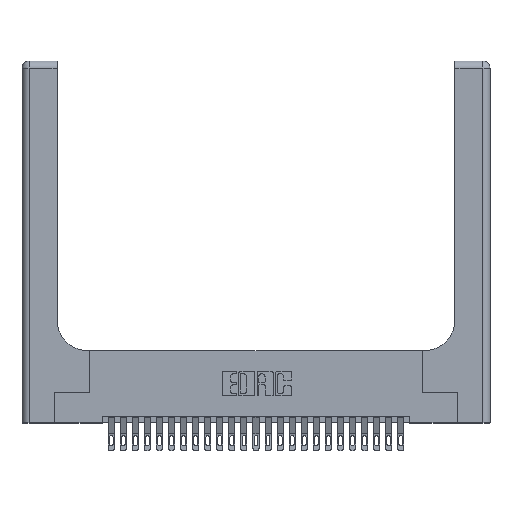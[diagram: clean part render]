
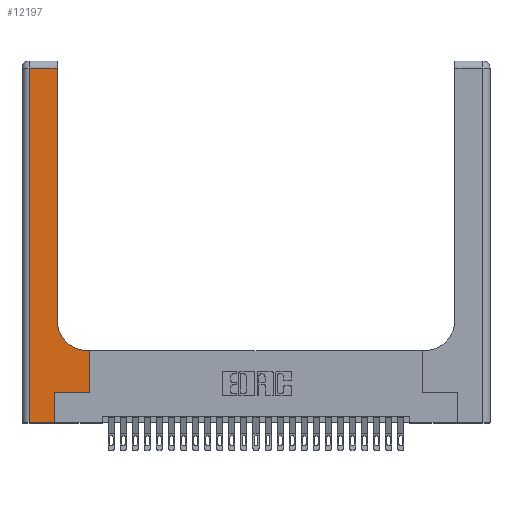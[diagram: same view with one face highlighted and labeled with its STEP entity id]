
A CAD part, top view. The second image highlights one B-rep face of the part: STEP entity #12197.
In plain terms, the highlighted planar face has unit normal (0, 0, 1).
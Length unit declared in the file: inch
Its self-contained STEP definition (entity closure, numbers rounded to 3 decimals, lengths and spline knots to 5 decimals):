
#12 = LINE ( 'NONE', #9352, #11336 ) ;
#282 = VERTEX_POINT ( 'NONE', #26497 ) ;
#387 = VERTEX_POINT ( 'NONE', #24511 ) ;
#941 = LINE ( 'NONE', #19317, #22839 ) ;
#1258 = DIRECTION ( 'NONE',  ( 0., 1., 0. ) ) ;
#1952 = ORIENTED_EDGE ( 'NONE', *, *, #21478, .T. ) ;
#2163 = VERTEX_POINT ( 'NONE', #24411 ) ;
#2564 = VECTOR ( 'NONE', #19264, 39.37008 ) ;
#2626 = CARTESIAN_POINT ( 'NONE',  ( 0.5585, 0.25, 0.37 ) ) ;
#2942 = EDGE_CURVE ( 'NONE', #15907, #387, #3555, .T. ) ;
#3529 = FACE_OUTER_BOUND ( 'NONE', #6134, .T. ) ;
#3555 = LINE ( 'NONE', #5350, #25381 ) ;
#3819 = CIRCLE ( 'NONE', #7777, 0.25 ) ;
#4368 = EDGE_CURVE ( 'NONE', #282, #26265, #15913, .T. ) ;
#5350 = CARTESIAN_POINT ( 'NONE',  ( 0.2915, 3., 0.37 ) ) ;
#5455 = CARTESIAN_POINT ( 'NONE',  ( 0., 2.94, 0.37 ) ) ;
#5601 = ORIENTED_EDGE ( 'NONE', *, *, #16830, .T. ) ;
#5917 = AXIS2_PLACEMENT_3D ( 'NONE', #23738, #25823, #13221 ) ;
#6134 = EDGE_LOOP ( 'NONE', ( #17461, #24082, #26692, #8557, #19874, #5601, #1952, #10276, #25451 ) ) ;
#7440 = DIRECTION ( 'NONE',  ( 1., 0., 0. ) ) ;
#7510 = CARTESIAN_POINT ( 'NONE',  ( 0.5415, 0.85, 0.37 ) ) ;
#7777 = AXIS2_PLACEMENT_3D ( 'NONE', #7510, #22324, #9649 ) ;
#7861 = CARTESIAN_POINT ( 'NONE',  ( 0.2915, 0.85, 0.37 ) ) ;
#8514 = EDGE_CURVE ( 'NONE', #19008, #24277, #12, .T. ) ;
#8557 = ORIENTED_EDGE ( 'NONE', *, *, #17998, .T. ) ;
#8939 = PLANE ( 'NONE',  #5917 ) ;
#9017 = CARTESIAN_POINT ( 'NONE',  ( 0.269, 0.25, 0.37 ) ) ;
#9352 = CARTESIAN_POINT ( 'NONE',  ( 0.2915, 0.6, 0.37 ) ) ;
#9645 = CARTESIAN_POINT ( 'NONE',  ( 0.06, 0., 0.37 ) ) ;
#9649 = DIRECTION ( 'NONE',  ( 1., 0., 0. ) ) ;
#10276 = ORIENTED_EDGE ( 'NONE', *, *, #8514, .T. ) ;
#10877 = DIRECTION ( 'NONE',  ( 1., 0., 0. ) ) ;
#11336 = VECTOR ( 'NONE', #11489, 39.37008 ) ;
#11489 = DIRECTION ( 'NONE',  ( -1., 0., 0. ) ) ;
#11527 = EDGE_CURVE ( 'NONE', #2163, #18370, #18841, .T. ) ;
#12197 = ADVANCED_FACE ( 'NONE', ( #3529 ), #8939, .F. ) ;
#12303 = VECTOR ( 'NONE', #17278, 39.37008 ) ;
#12411 = CARTESIAN_POINT ( 'NONE',  ( 0.06, 3., 0.37 ) ) ;
#13221 = DIRECTION ( 'NONE',  ( -1., 0., 0. ) ) ;
#13925 = DIRECTION ( 'NONE',  ( -1., 0., 0. ) ) ;
#15057 = VECTOR ( 'NONE', #13925, 39.37008 ) ;
#15148 = CARTESIAN_POINT ( 'NONE',  ( 0.5585, 0.25, 0.37 ) ) ;
#15493 = CARTESIAN_POINT ( 'NONE',  ( 0.5585, 0.6, 0.37 ) ) ;
#15907 = VERTEX_POINT ( 'NONE', #7861 ) ;
#15913 = LINE ( 'NONE', #12411, #25751 ) ;
#16830 = EDGE_CURVE ( 'NONE', #18370, #19606, #941, .T. ) ;
#17278 = DIRECTION ( 'NONE',  ( 0., 1., 0. ) ) ;
#17461 = ORIENTED_EDGE ( 'NONE', *, *, #2942, .T. ) ;
#17998 = EDGE_CURVE ( 'NONE', #26265, #2163, #25015, .T. ) ;
#18370 = VERTEX_POINT ( 'NONE', #9017 ) ;
#18546 = EDGE_CURVE ( 'NONE', #24277, #15907, #3819, .T. ) ;
#18841 = LINE ( 'NONE', #25569, #2564 ) ;
#19008 = VERTEX_POINT ( 'NONE', #15493 ) ;
#19264 = DIRECTION ( 'NONE',  ( 0., 1., 0. ) ) ;
#19317 = CARTESIAN_POINT ( 'NONE',  ( 0.269, 0.25, 0.37 ) ) ;
#19599 = CARTESIAN_POINT ( 'NONE',  ( 0.5415, 0.6, 0.37 ) ) ;
#19606 = VERTEX_POINT ( 'NONE', #2626 ) ;
#19874 = ORIENTED_EDGE ( 'NONE', *, *, #11527, .T. ) ;
#20005 = EDGE_CURVE ( 'NONE', #387, #282, #26249, .T. ) ;
#21478 = EDGE_CURVE ( 'NONE', #19606, #19008, #24209, .T. ) ;
#22254 = CARTESIAN_POINT ( 'NONE',  ( 0., 0., 0.37 ) ) ;
#22324 = DIRECTION ( 'NONE',  ( 0., 0., -1. ) ) ;
#22839 = VECTOR ( 'NONE', #10877, 39.37008 ) ;
#23738 = CARTESIAN_POINT ( 'NONE',  ( 0., 3., 0.37 ) ) ;
#24082 = ORIENTED_EDGE ( 'NONE', *, *, #20005, .T. ) ;
#24209 = LINE ( 'NONE', #15148, #12303 ) ;
#24277 = VERTEX_POINT ( 'NONE', #19599 ) ;
#24411 = CARTESIAN_POINT ( 'NONE',  ( 0.269, 0., 0.37 ) ) ;
#24511 = CARTESIAN_POINT ( 'NONE',  ( 0.2915, 2.94, 0.37 ) ) ;
#25015 = LINE ( 'NONE', #22254, #25647 ) ;
#25381 = VECTOR ( 'NONE', #1258, 39.37008 ) ;
#25451 = ORIENTED_EDGE ( 'NONE', *, *, #18546, .T. ) ;
#25569 = CARTESIAN_POINT ( 'NONE',  ( 0.269, 0., 0.37 ) ) ;
#25647 = VECTOR ( 'NONE', #7440, 39.37008 ) ;
#25751 = VECTOR ( 'NONE', #27170, 39.37008 ) ;
#25823 = DIRECTION ( 'NONE',  ( 0., 0., -1. ) ) ;
#26249 = LINE ( 'NONE', #5455, #15057 ) ;
#26265 = VERTEX_POINT ( 'NONE', #9645 ) ;
#26497 = CARTESIAN_POINT ( 'NONE',  ( 0.06, 2.94, 0.37 ) ) ;
#26692 = ORIENTED_EDGE ( 'NONE', *, *, #4368, .T. ) ;
#27170 = DIRECTION ( 'NONE',  ( 0., -1., 0. ) ) ;
